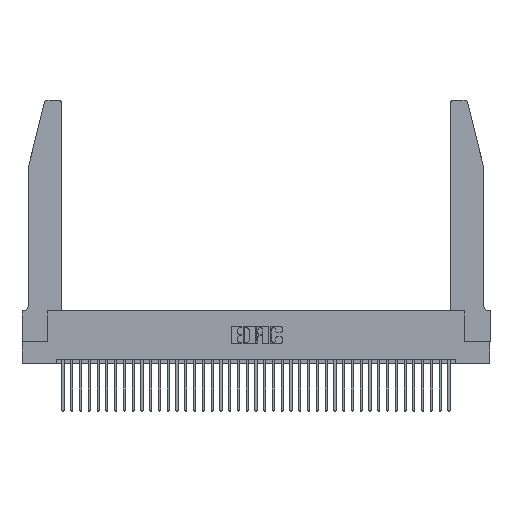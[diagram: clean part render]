
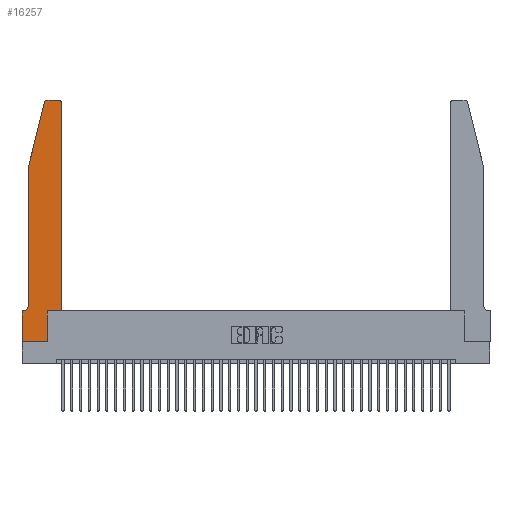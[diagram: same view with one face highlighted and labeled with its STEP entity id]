
A CAD part, top view. The second image highlights one B-rep face of the part: STEP entity #16257.
In plain terms, the highlighted planar face has unit normal (0, 0, 1).
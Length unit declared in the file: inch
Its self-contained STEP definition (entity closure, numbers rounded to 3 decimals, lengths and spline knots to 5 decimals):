
#1119 = EDGE_CURVE ( 'NONE', #17309, #26350, #13791, .T. ) ;
#1544 = ORIENTED_EDGE ( 'NONE', *, *, #12925, .T. ) ;
#2032 = VERTEX_POINT ( 'NONE', #29536 ) ;
#2503 = CARTESIAN_POINT ( 'NONE',  ( 0.0755, 2., 0.37 ) ) ;
#2706 = CARTESIAN_POINT ( 'NONE',  ( 0.0755, 2., 0.37 ) ) ;
#2934 = LINE ( 'NONE', #13405, #9449 ) ;
#3118 = DIRECTION ( 'NONE',  ( 1., 0., 0. ) ) ;
#3280 = ORIENTED_EDGE ( 'NONE', *, *, #31574, .T. ) ;
#3804 = ORIENTED_EDGE ( 'NONE', *, *, #28761, .T. ) ;
#4277 = ORIENTED_EDGE ( 'NONE', *, *, #38216, .T. ) ;
#4386 = EDGE_CURVE ( 'NONE', #18414, #2032, #11083, .T. ) ;
#4844 = DIRECTION ( 'NONE',  ( 0., 0., 1. ) ) ;
#5364 = VECTOR ( 'NONE', #19700, 39.37008 ) ;
#5905 = CARTESIAN_POINT ( 'NONE',  ( 0., 0.35, 0.37 ) ) ;
#6444 = CARTESIAN_POINT ( 'NONE',  ( 0.2865, 0., 0.37 ) ) ;
#7062 = LINE ( 'NONE', #2706, #22506 ) ;
#7169 = AXIS2_PLACEMENT_3D ( 'NONE', #23346, #4844, #26347 ) ;
#7770 = DIRECTION ( 'NONE',  ( 0., 1., 0. ) ) ;
#8079 = VECTOR ( 'NONE', #13933, 39.37008 ) ;
#8405 = CARTESIAN_POINT ( 'NONE',  ( 0.4205, 2.75, 0.37 ) ) ;
#9449 = VECTOR ( 'NONE', #16491, 39.37008 ) ;
#9736 = ORIENTED_EDGE ( 'NONE', *, *, #25276, .T. ) ;
#10449 = CARTESIAN_POINT ( 'NONE',  ( 0., 0., 0.37 ) ) ;
#10795 = CARTESIAN_POINT ( 'NONE',  ( 0.4505, 0.35, 0.37 ) ) ;
#11083 = CIRCLE ( 'NONE', #18435, 0.03 ) ;
#11520 = CARTESIAN_POINT ( 'NONE',  ( 0., 0.35, 0.37 ) ) ;
#12177 = EDGE_CURVE ( 'NONE', #14906, #17309, #2934, .T. ) ;
#12292 = VERTEX_POINT ( 'NONE', #35715 ) ;
#12925 = EDGE_CURVE ( 'NONE', #19033, #18414, #16199, .T. ) ;
#13050 = CARTESIAN_POINT ( 'NONE',  ( 0.0755, 2., 0.37 ) ) ;
#13405 = CARTESIAN_POINT ( 'NONE',  ( 0., 0., 0.37 ) ) ;
#13791 = LINE ( 'NONE', #10449, #5364 ) ;
#13933 = DIRECTION ( 'NONE',  ( 0., 1., 0. ) ) ;
#14061 = FACE_OUTER_BOUND ( 'NONE', #20128, .T. ) ;
#14270 = ORIENTED_EDGE ( 'NONE', *, *, #17578, .T. ) ;
#14649 = DIRECTION ( 'NONE',  ( 0., 0., 1. ) ) ;
#14906 = VERTEX_POINT ( 'NONE', #5905 ) ;
#14930 = LINE ( 'NONE', #23618, #29890 ) ;
#15142 = CARTESIAN_POINT ( 'NONE',  ( 0.0755, 0.42, 0.37 ) ) ;
#15939 = VERTEX_POINT ( 'NONE', #13050 ) ;
#16199 = LINE ( 'NONE', #38341, #31140 ) ;
#16256 = VECTOR ( 'NONE', #7770, 39.37008 ) ;
#16257 = ADVANCED_FACE ( 'NONE', ( #14061 ), #29574, .T. ) ;
#16491 = DIRECTION ( 'NONE',  ( 0., -1., 0. ) ) ;
#16687 = ORIENTED_EDGE ( 'NONE', *, *, #1119, .T. ) ;
#17309 = VERTEX_POINT ( 'NONE', #24952 ) ;
#17351 = CARTESIAN_POINT ( 'NONE',  ( 0.4505, 2.72, 0.37 ) ) ;
#17578 = EDGE_CURVE ( 'NONE', #25694, #14906, #14930, .T. ) ;
#18094 = CARTESIAN_POINT ( 'NONE',  ( 0.0055, 0.42, 0.37 ) ) ;
#18414 = VERTEX_POINT ( 'NONE', #29307 ) ;
#18435 = AXIS2_PLACEMENT_3D ( 'NONE', #39669, #21750, #3118 ) ;
#18462 = DIRECTION ( 'NONE',  ( -0.239, -0.971, 0. ) ) ;
#19033 = VERTEX_POINT ( 'NONE', #8405 ) ;
#19350 = CIRCLE ( 'NONE', #7169, 0.03 ) ;
#19462 = DIRECTION ( 'NONE',  ( 1., 0., 0. ) ) ;
#19662 = VECTOR ( 'NONE', #19462, 39.37008 ) ;
#19700 = DIRECTION ( 'NONE',  ( 1., 0., 0. ) ) ;
#20128 = EDGE_LOOP ( 'NONE', ( #1544, #28118, #3280, #3804, #38145, #14270, #39637, #16687, #32928, #4277, #30595, #9736 ) ) ;
#21133 = DIRECTION ( 'NONE',  ( -1., 0., 0. ) ) ;
#21309 = DIRECTION ( 'NONE',  ( 0., -1., 0. ) ) ;
#21750 = DIRECTION ( 'NONE',  ( 0., 0., 1. ) ) ;
#22506 = VECTOR ( 'NONE', #18462, 39.37008 ) ;
#22912 = CARTESIAN_POINT ( 'NONE',  ( 0.4505, 0.35, 0.37 ) ) ;
#23346 = CARTESIAN_POINT ( 'NONE',  ( 0.4205, 2.72, 0.37 ) ) ;
#23366 = AXIS2_PLACEMENT_3D ( 'NONE', #18094, #39034, #21133 ) ;
#23431 = DIRECTION ( 'NONE',  ( -1., 0., 0. ) ) ;
#23618 = CARTESIAN_POINT ( 'NONE',  ( 0.0755, 0.35, 0.37 ) ) ;
#23777 = EDGE_CURVE ( 'NONE', #37876, #25694, #24550, .T. ) ;
#24220 = LINE ( 'NONE', #29084, #16256 ) ;
#24253 = VECTOR ( 'NONE', #21309, 39.37008 ) ;
#24550 = CIRCLE ( 'NONE', #23366, 0.07 ) ;
#24952 = CARTESIAN_POINT ( 'NONE',  ( 0., 0., 0.37 ) ) ;
#25276 = EDGE_CURVE ( 'NONE', #36315, #19033, #19350, .T. ) ;
#25694 = VERTEX_POINT ( 'NONE', #31115 ) ;
#26347 = DIRECTION ( 'NONE',  ( 1., 0., 0. ) ) ;
#26350 = VERTEX_POINT ( 'NONE', #6444 ) ;
#26617 = DIRECTION ( 'NONE',  ( -1., 0., 0. ) ) ;
#28118 = ORIENTED_EDGE ( 'NONE', *, *, #4386, .T. ) ;
#28452 = CARTESIAN_POINT ( 'NONE',  ( 0.4505, 0.35, 0.37 ) ) ;
#28761 = EDGE_CURVE ( 'NONE', #15939, #37876, #32171, .T. ) ;
#29084 = CARTESIAN_POINT ( 'NONE',  ( 0.2865, 0.35, 0.37 ) ) ;
#29212 = EDGE_CURVE ( 'NONE', #26350, #12292, #24220, .T. ) ;
#29307 = CARTESIAN_POINT ( 'NONE',  ( 0.284, 2.75, 0.37 ) ) ;
#29536 = CARTESIAN_POINT ( 'NONE',  ( 0.25487, 2.72718, 0.37 ) ) ;
#29574 = PLANE ( 'NONE',  #29698 ) ;
#29698 = AXIS2_PLACEMENT_3D ( 'NONE', #11520, #14649, #35573 ) ;
#29874 = VERTEX_POINT ( 'NONE', #22912 ) ;
#29890 = VECTOR ( 'NONE', #26617, 39.37008 ) ;
#30595 = ORIENTED_EDGE ( 'NONE', *, *, #37600, .T. ) ;
#31115 = CARTESIAN_POINT ( 'NONE',  ( 0.0055, 0.35, 0.37 ) ) ;
#31140 = VECTOR ( 'NONE', #23431, 39.37008 ) ;
#31574 = EDGE_CURVE ( 'NONE', #2032, #15939, #7062, .T. ) ;
#32171 = LINE ( 'NONE', #2503, #24253 ) ;
#32278 = LINE ( 'NONE', #10795, #8079 ) ;
#32928 = ORIENTED_EDGE ( 'NONE', *, *, #29212, .T. ) ;
#34567 = LINE ( 'NONE', #28452, #19662 ) ;
#35573 = DIRECTION ( 'NONE',  ( 1., 0., 0. ) ) ;
#35715 = CARTESIAN_POINT ( 'NONE',  ( 0.2865, 0.35, 0.37 ) ) ;
#36315 = VERTEX_POINT ( 'NONE', #17351 ) ;
#37600 = EDGE_CURVE ( 'NONE', #29874, #36315, #32278, .T. ) ;
#37876 = VERTEX_POINT ( 'NONE', #15142 ) ;
#38145 = ORIENTED_EDGE ( 'NONE', *, *, #23777, .T. ) ;
#38216 = EDGE_CURVE ( 'NONE', #12292, #29874, #34567, .T. ) ;
#38341 = CARTESIAN_POINT ( 'NONE',  ( 0.2605, 2.75, 0.37 ) ) ;
#39034 = DIRECTION ( 'NONE',  ( 0., 0., -1. ) ) ;
#39637 = ORIENTED_EDGE ( 'NONE', *, *, #12177, .T. ) ;
#39669 = CARTESIAN_POINT ( 'NONE',  ( 0.284, 2.72, 0.37 ) ) ;
